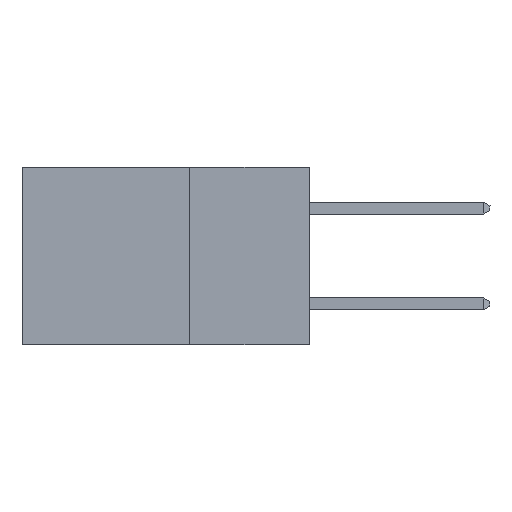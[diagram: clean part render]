
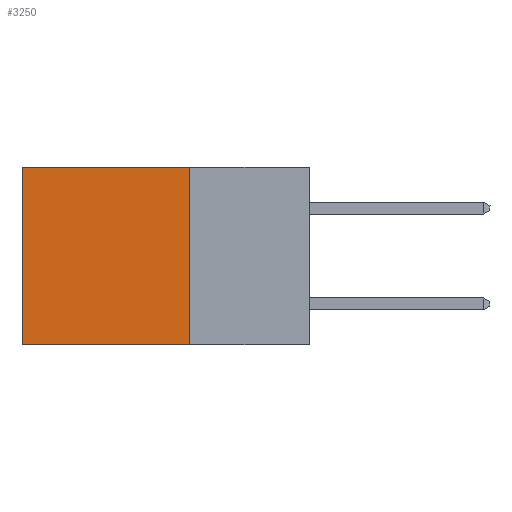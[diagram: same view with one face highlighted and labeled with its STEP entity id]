
A CAD part, left-side view. The second image highlights one B-rep face of the part: STEP entity #3250.
In plain terms, the highlighted planar face has unit normal (-1, 0, 0).
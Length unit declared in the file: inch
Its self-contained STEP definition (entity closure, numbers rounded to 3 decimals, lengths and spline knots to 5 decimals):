
#355 = DIRECTION ( 'NONE',  ( 0., 1., 0. ) ) ;
#925 = LINE ( 'NONE', #10399, #13971 ) ;
#1947 = VERTEX_POINT ( 'NONE', #13632 ) ;
#2902 = FACE_OUTER_BOUND ( 'NONE', #11694, .T. ) ;
#3190 = VERTEX_POINT ( 'NONE', #15170 ) ;
#3250 = ADVANCED_FACE ( 'NONE', ( #2902 ), #14548, .F. ) ;
#3593 = EDGE_CURVE ( 'NONE', #7208, #3190, #10911, .T. ) ;
#3651 = VECTOR ( 'NONE', #12941, 39.37008 ) ;
#5216 = CARTESIAN_POINT ( 'NONE',  ( 0.2875, 0.6, -0.37 ) ) ;
#5458 = ORIENTED_EDGE ( 'NONE', *, *, #14702, .F. ) ;
#6687 = EDGE_CURVE ( 'NONE', #3190, #11652, #13889, .T. ) ;
#7208 = VERTEX_POINT ( 'NONE', #12584 ) ;
#7711 = VECTOR ( 'NONE', #10191, 39.37008 ) ;
#9268 = DIRECTION ( 'NONE',  ( 0., 0., -1. ) ) ;
#10191 = DIRECTION ( 'NONE',  ( 0., 1., 0. ) ) ;
#10364 = CARTESIAN_POINT ( 'NONE',  ( 0.2875, 0.25, 0. ) ) ;
#10399 = CARTESIAN_POINT ( 'NONE',  ( 0.2875, 0.25, 0. ) ) ;
#10911 = LINE ( 'NONE', #10364, #7711 ) ;
#11652 = VERTEX_POINT ( 'NONE', #5216 ) ;
#11694 = EDGE_LOOP ( 'NONE', ( #13947, #5458, #14812, #12904 ) ) ;
#12584 = CARTESIAN_POINT ( 'NONE',  ( 0.2875, 0.25, 0. ) ) ;
#12904 = ORIENTED_EDGE ( 'NONE', *, *, #3593, .T. ) ;
#12941 = DIRECTION ( 'NONE',  ( 0., 0., -1. ) ) ;
#13108 = CARTESIAN_POINT ( 'NONE',  ( 0.2875, 0.25, -0.37 ) ) ;
#13131 = VECTOR ( 'NONE', #355, 39.37008 ) ;
#13632 = CARTESIAN_POINT ( 'NONE',  ( 0.2875, 0.25, -0.37 ) ) ;
#13889 = LINE ( 'NONE', #14018, #3651 ) ;
#13947 = ORIENTED_EDGE ( 'NONE', *, *, #6687, .T. ) ;
#13971 = VECTOR ( 'NONE', #9268, 39.37008 ) ;
#14018 = CARTESIAN_POINT ( 'NONE',  ( 0.2875, 0.6, 0. ) ) ;
#14531 = DIRECTION ( 'NONE',  ( 0., 0., -1. ) ) ;
#14548 = PLANE ( 'NONE',  #14617 ) ;
#14596 = CARTESIAN_POINT ( 'NONE',  ( 0.2875, 0.25, 0. ) ) ;
#14617 = AXIS2_PLACEMENT_3D ( 'NONE', #14596, #14668, #14531 ) ;
#14668 = DIRECTION ( 'NONE',  ( 1., 0., 0. ) ) ;
#14702 = EDGE_CURVE ( 'NONE', #1947, #11652, #16053, .T. ) ;
#14812 = ORIENTED_EDGE ( 'NONE', *, *, #15793, .F. ) ;
#15170 = CARTESIAN_POINT ( 'NONE',  ( 0.2875, 0.6, 0. ) ) ;
#15793 = EDGE_CURVE ( 'NONE', #7208, #1947, #925, .T. ) ;
#16053 = LINE ( 'NONE', #13108, #13131 ) ;
